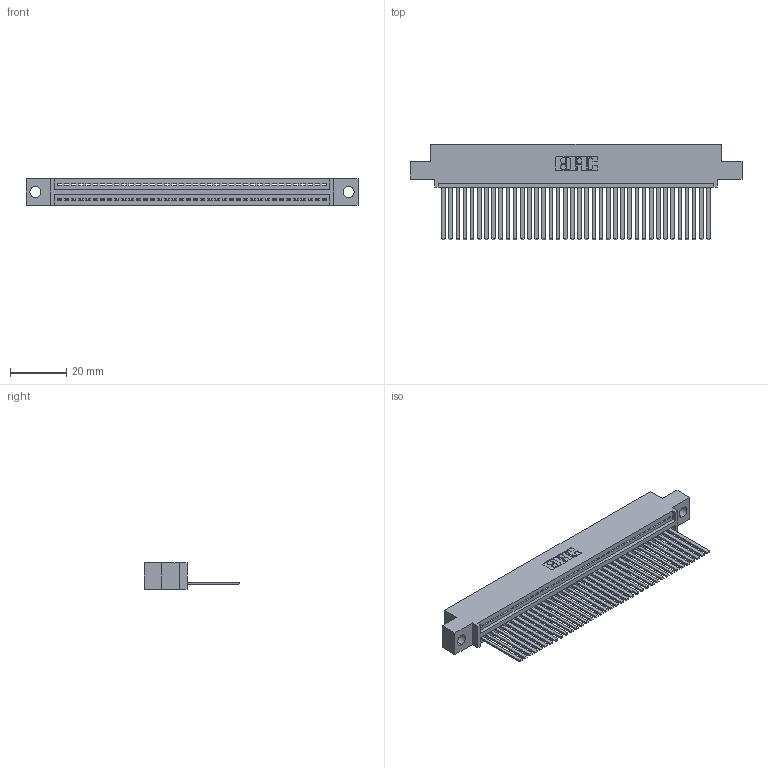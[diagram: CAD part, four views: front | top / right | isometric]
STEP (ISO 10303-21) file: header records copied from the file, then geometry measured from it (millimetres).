
FILE_DESCRIPTION (( 'STEP AP203' ), '1' );
FILE_NAME ('395-038-544-404.STEP', '2018-11-14T05:21:13', ( '' ), ( '' ), 'SwSTEP 2.0', 'SolidWorks 2016', '' );
FILE_SCHEMA (( 'CONFIG_CONTROL_DESIGN' ));
Length unit declared in the file: inch
Products named in the file (3): 395-038-544-404; 345 Part_0.110 Offset - 0.156 Dia-TH; 345-292-001_345-293-144
Assembly tree (39 placements, depth 2):
  395-038-544-404
    345 Part_0.110 Offset - 0.156 Dia-TH
    345-292-001_345-293-144  x38
Bounding box: 117.73 x 33.96 x 9.4 mm (x, y, z)
Volume: 11428.1 mm3; surface area: 16344.4 mm2
Topology: 39 solids, 39 shells, 2106 faces, 6357 edges, 4186 vertices
Faces by surface type: plane 1452, cylinder 654
Entity records: 29089 total; most frequent: CARTESIAN_POINT 5046, ORIENTED_EDGE 5018, DIRECTION 4409, EDGE_CURVE 2509, VECTOR 2229, LINE 2229, VERTEX_POINT 1670, AXIS2_PLACEMENT_3D 1090
